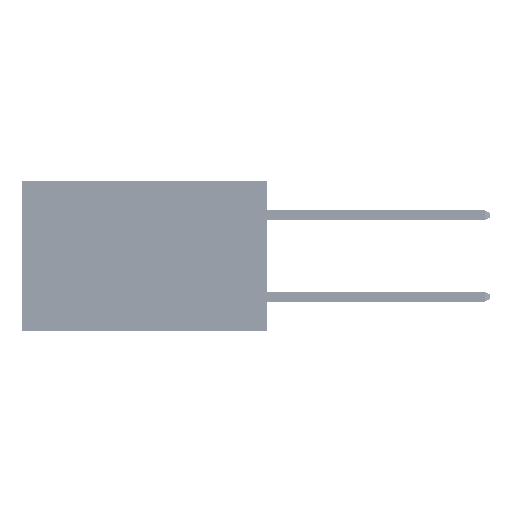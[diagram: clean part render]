
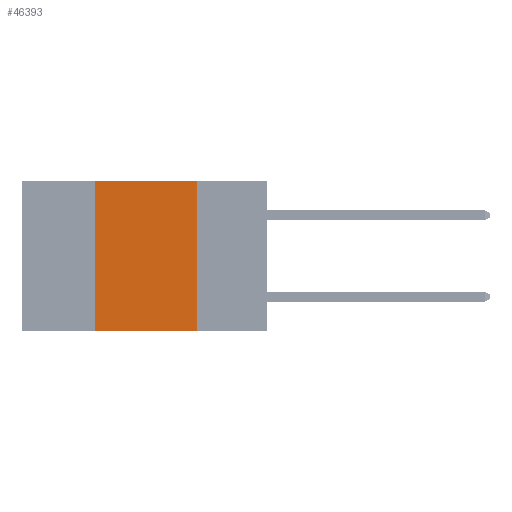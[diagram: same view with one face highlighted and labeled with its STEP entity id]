
A CAD part, left-side view. The second image highlights one B-rep face of the part: STEP entity #46393.
In plain terms, the highlighted planar face has unit normal (-1, 0, 0).
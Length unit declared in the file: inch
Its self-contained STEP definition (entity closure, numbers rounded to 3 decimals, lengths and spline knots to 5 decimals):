
#820 = VERTEX_POINT ( 'NONE', #1633 ) ;
#1505 = LINE ( 'NONE', #12467, #19231 ) ;
#1633 = CARTESIAN_POINT ( 'NONE',  ( 0., 0.17, -0.37 ) ) ;
#3498 = ORIENTED_EDGE ( 'NONE', *, *, #34268, .F. ) ;
#4494 = VERTEX_POINT ( 'NONE', #34866 ) ;
#5001 = LINE ( 'NONE', #12225, #9528 ) ;
#5980 = EDGE_LOOP ( 'NONE', ( #8474, #12550, #3498, #40955 ) ) ;
#8152 = VECTOR ( 'NONE', #47332, 39.37008 ) ;
#8474 = ORIENTED_EDGE ( 'NONE', *, *, #43477, .F. ) ;
#9528 = VECTOR ( 'NONE', #47080, 39.37008 ) ;
#10583 = CARTESIAN_POINT ( 'NONE',  ( 0., 0.42, 0. ) ) ;
#12225 = CARTESIAN_POINT ( 'NONE',  ( 0., 0.6, -0.37 ) ) ;
#12467 = CARTESIAN_POINT ( 'NONE',  ( 0., 0.6, 0. ) ) ;
#12550 = ORIENTED_EDGE ( 'NONE', *, *, #33044, .F. ) ;
#13330 = DIRECTION ( 'NONE',  ( 0., 0., -1. ) ) ;
#14807 = DIRECTION ( 'NONE',  ( 0., 0., 1. ) ) ;
#16205 = VERTEX_POINT ( 'NONE', #34582 ) ;
#16557 = CARTESIAN_POINT ( 'NONE',  ( 0., 0.6, 0. ) ) ;
#19231 = VECTOR ( 'NONE', #42590, 39.37008 ) ;
#19867 = VECTOR ( 'NONE', #14807, 39.37008 ) ;
#24503 = PLANE ( 'NONE',  #27409 ) ;
#27409 = AXIS2_PLACEMENT_3D ( 'NONE', #16557, #31981, #13330 ) ;
#29430 = CARTESIAN_POINT ( 'NONE',  ( 0., 0.42, 0. ) ) ;
#31981 = DIRECTION ( 'NONE',  ( 1., 0., 0. ) ) ;
#32597 = LINE ( 'NONE', #47091, #8152 ) ;
#33044 = EDGE_CURVE ( 'NONE', #36068, #4494, #1505, .T. ) ;
#33199 = LINE ( 'NONE', #10583, #19867 ) ;
#34268 = EDGE_CURVE ( 'NONE', #16205, #36068, #33199, .T. ) ;
#34582 = CARTESIAN_POINT ( 'NONE',  ( 0., 0.42, -0.37 ) ) ;
#34866 = CARTESIAN_POINT ( 'NONE',  ( 0., 0.17, 0. ) ) ;
#36068 = VERTEX_POINT ( 'NONE', #29430 ) ;
#36215 = FACE_OUTER_BOUND ( 'NONE', #5980, .T. ) ;
#38761 = EDGE_CURVE ( 'NONE', #16205, #820, #5001, .T. ) ;
#40955 = ORIENTED_EDGE ( 'NONE', *, *, #38761, .T. ) ;
#42590 = DIRECTION ( 'NONE',  ( 0., -1., 0. ) ) ;
#43477 = EDGE_CURVE ( 'NONE', #4494, #820, #32597, .T. ) ;
#46393 = ADVANCED_FACE ( 'NONE', ( #36215 ), #24503, .F. ) ;
#47080 = DIRECTION ( 'NONE',  ( 0., -1., 0. ) ) ;
#47091 = CARTESIAN_POINT ( 'NONE',  ( 0., 0.17, 0. ) ) ;
#47332 = DIRECTION ( 'NONE',  ( 0., 0., -1. ) ) ;
